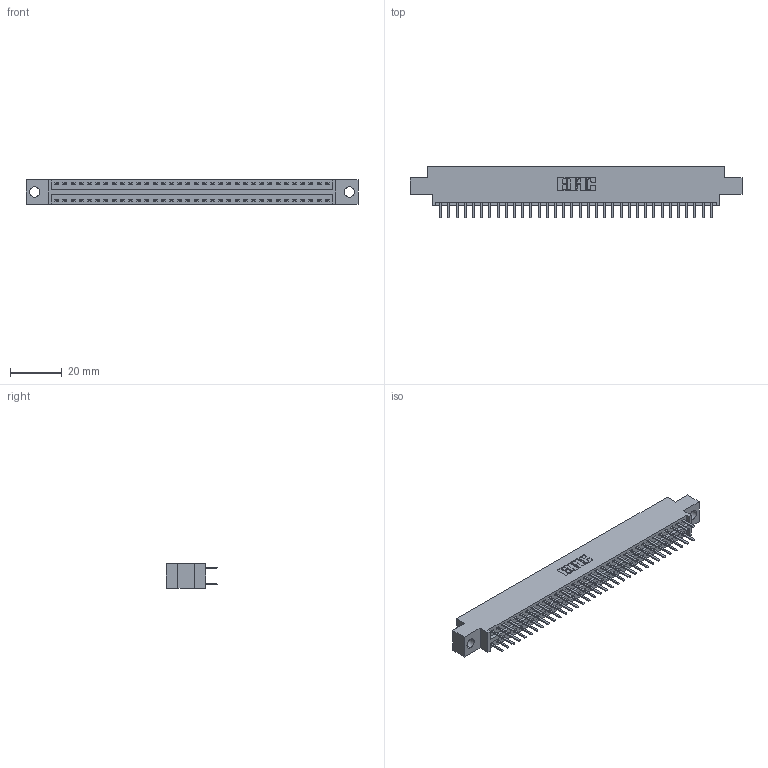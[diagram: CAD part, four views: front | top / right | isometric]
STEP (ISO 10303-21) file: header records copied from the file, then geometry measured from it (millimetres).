
FILE_DESCRIPTION (( 'STEP AP203' ), '1' );
FILE_NAME ('396-068-520-804.STEP', '2018-09-08T20:44:00', ( '' ), ( '' ), 'SwSTEP 2.0', 'SolidWorks 2016', '' );
FILE_SCHEMA (( 'CONFIG_CONTROL_DESIGN' ));
Length unit declared in the file: inch
Products named in the file (3): 346 Part_0.170 Offset - 0.156 Dia-TH; 345-292-001_345-293-120; 396-068-520-804
Assembly tree (69 placements, depth 2):
  396-068-520-804
    346 Part_0.170 Offset - 0.156 Dia-TH
    345-292-001_345-293-120  x68
Bounding box: 128.52 x 20.02 x 9.4 mm (x, y, z)
Volume: 12198.2 mm3; surface area: 16564.4 mm2
Topology: 69 solids, 69 shells, 3934 faces, 11425 edges, 7434 vertices
Faces by surface type: plane 2596, cylinder 1338
Entity records: 23515 total; most frequent: CARTESIAN_POINT 3900, ORIENTED_EDGE 3822, DIRECTION 3475, EDGE_CURVE 1911, VECTOR 1639, LINE 1639, VERTEX_POINT 1270, AXIS2_PLACEMENT_3D 918
